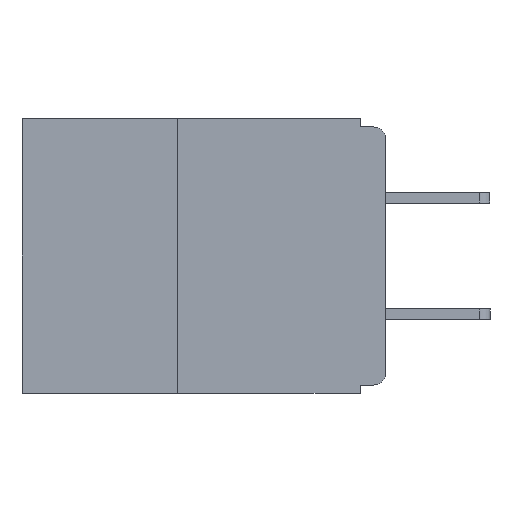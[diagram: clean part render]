
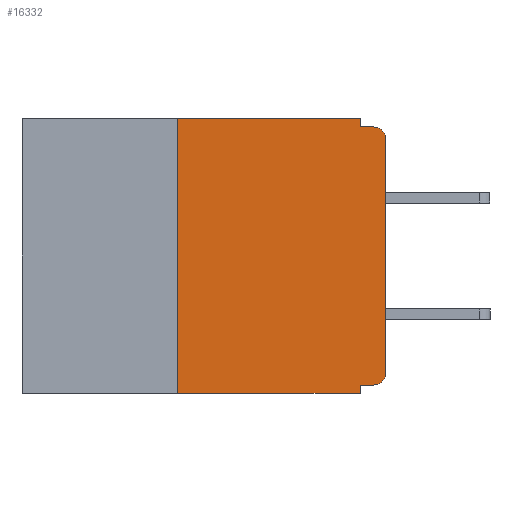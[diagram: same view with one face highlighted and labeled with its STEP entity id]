
A CAD part, left-side view. The second image highlights one B-rep face of the part: STEP entity #16332.
In plain terms, the highlighted planar face has unit normal (-1, 0, 0).
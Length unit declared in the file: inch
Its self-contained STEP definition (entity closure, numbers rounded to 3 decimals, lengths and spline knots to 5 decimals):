
#47 = VERTEX_POINT ( 'NONE', #5256 ) ;
#73 = VECTOR ( 'NONE', #1274, 39.37008 ) ;
#416 = ORIENTED_EDGE ( 'NONE', *, *, #1629, .F. ) ;
#909 = EDGE_CURVE ( 'NONE', #18240, #13265, #12853, .T. ) ;
#1192 = DIRECTION ( 'NONE',  ( 0., 0., 1. ) ) ;
#1197 = VERTEX_POINT ( 'NONE', #9864 ) ;
#1203 = LINE ( 'NONE', #15534, #5566 ) ;
#1274 = DIRECTION ( 'NONE',  ( 0., 0., -1. ) ) ;
#1463 = DIRECTION ( 'NONE',  ( 0., 0., -1. ) ) ;
#1629 = EDGE_CURVE ( 'NONE', #2551, #6083, #1203, .T. ) ;
#1816 = CARTESIAN_POINT ( 'NONE',  ( 0., 0.031, 0. ) ) ;
#2259 = CARTESIAN_POINT ( 'NONE',  ( 0., 0.437, 0. ) ) ;
#2526 = CARTESIAN_POINT ( 'NONE',  ( 0., 0.437, -0.33 ) ) ;
#2551 = VERTEX_POINT ( 'NONE', #12666 ) ;
#2767 = ORIENTED_EDGE ( 'NONE', *, *, #18670, .F. ) ;
#2886 = VECTOR ( 'NONE', #13590, 39.37008 ) ;
#2897 = CARTESIAN_POINT ( 'NONE',  ( 0., 0., 0. ) ) ;
#3027 = DIRECTION ( 'NONE',  ( -1., 0., 0. ) ) ;
#3041 = ORIENTED_EDGE ( 'NONE', *, *, #909, .F. ) ;
#3880 = EDGE_CURVE ( 'NONE', #14055, #14395, #18166, .T. ) ;
#3926 = DIRECTION ( 'NONE',  ( 0., 0., -1. ) ) ;
#4082 = CARTESIAN_POINT ( 'NONE',  ( 0., 0.437, 0. ) ) ;
#4648 = CARTESIAN_POINT ( 'NONE',  ( 0., 0.015, -0.025 ) ) ;
#4887 = AXIS2_PLACEMENT_3D ( 'NONE', #2259, #13332, #3926 ) ;
#5198 = EDGE_LOOP ( 'NONE', ( #14448, #10715, #2767, #12185, #20731, #416, #17470, #3041, #16209, #5558 ) ) ;
#5256 = CARTESIAN_POINT ( 'NONE',  ( 0., 0., -0.305 ) ) ;
#5280 = CARTESIAN_POINT ( 'NONE',  ( 0., 0., -0.01 ) ) ;
#5324 = EDGE_CURVE ( 'NONE', #2551, #13265, #7125, .T. ) ;
#5431 = LINE ( 'NONE', #2897, #16574 ) ;
#5490 = VECTOR ( 'NONE', #1463, 39.37008 ) ;
#5558 = ORIENTED_EDGE ( 'NONE', *, *, #18409, .T. ) ;
#5566 = VECTOR ( 'NONE', #15554, 39.37008 ) ;
#5738 = CARTESIAN_POINT ( 'NONE',  ( 0., 0.015, -0.32 ) ) ;
#5765 = CARTESIAN_POINT ( 'NONE',  ( 0., 0.031, -0.32 ) ) ;
#5852 = FACE_OUTER_BOUND ( 'NONE', #5198, .T. ) ;
#6083 = VERTEX_POINT ( 'NONE', #15545 ) ;
#6241 = DIRECTION ( 'NONE',  ( 0., 0., -1. ) ) ;
#6377 = VECTOR ( 'NONE', #20636, 39.37008 ) ;
#6525 = AXIS2_PLACEMENT_3D ( 'NONE', #4648, #15711, #6241 ) ;
#7125 = LINE ( 'NONE', #2526, #2886 ) ;
#8442 = DIRECTION ( 'NONE',  ( 0., -1., 0. ) ) ;
#9452 = CIRCLE ( 'NONE', #6525, 0.015 ) ;
#9468 = EDGE_CURVE ( 'NONE', #17992, #1197, #9452, .T. ) ;
#9864 = CARTESIAN_POINT ( 'NONE',  ( 0., 0.015, -0.01 ) ) ;
#10715 = ORIENTED_EDGE ( 'NONE', *, *, #9468, .T. ) ;
#10950 = CARTESIAN_POINT ( 'NONE',  ( 0., 0.031, -0.33 ) ) ;
#11063 = CARTESIAN_POINT ( 'NONE',  ( 0., 0., -0.32 ) ) ;
#12185 = ORIENTED_EDGE ( 'NONE', *, *, #3880, .F. ) ;
#12259 = CARTESIAN_POINT ( 'NONE',  ( 0., 0.031, -0.01 ) ) ;
#12495 = CARTESIAN_POINT ( 'NONE',  ( 0., 0.015, -0.305 ) ) ;
#12666 = CARTESIAN_POINT ( 'NONE',  ( 0., 0.25, -0.33 ) ) ;
#12853 = LINE ( 'NONE', #16391, #73 ) ;
#12930 = VECTOR ( 'NONE', #16735, 39.37008 ) ;
#13131 = VECTOR ( 'NONE', #8442, 39.37008 ) ;
#13265 = VERTEX_POINT ( 'NONE', #10950 ) ;
#13332 = DIRECTION ( 'NONE',  ( 1., 0., 0. ) ) ;
#13590 = DIRECTION ( 'NONE',  ( 0., -1., 0. ) ) ;
#14055 = VERTEX_POINT ( 'NONE', #19525 ) ;
#14105 = DIRECTION ( 'NONE',  ( 0., 0., -1. ) ) ;
#14310 = VERTEX_POINT ( 'NONE', #5738 ) ;
#14395 = VERTEX_POINT ( 'NONE', #12259 ) ;
#14448 = ORIENTED_EDGE ( 'NONE', *, *, #15033, .T. ) ;
#14848 = AXIS2_PLACEMENT_3D ( 'NONE', #12495, #3027, #14105 ) ;
#15033 = EDGE_CURVE ( 'NONE', #47, #17992, #5431, .T. ) ;
#15534 = CARTESIAN_POINT ( 'NONE',  ( 0., 0.25, -0.33 ) ) ;
#15545 = CARTESIAN_POINT ( 'NONE',  ( 0., 0.25, 0. ) ) ;
#15554 = DIRECTION ( 'NONE',  ( 0., 0., 1. ) ) ;
#15711 = DIRECTION ( 'NONE',  ( -1., 0., 0. ) ) ;
#15836 = EDGE_CURVE ( 'NONE', #14310, #18240, #19057, .T. ) ;
#16209 = ORIENTED_EDGE ( 'NONE', *, *, #15836, .F. ) ;
#16332 = ADVANCED_FACE ( 'NONE', ( #5852 ), #19688, .F. ) ;
#16391 = CARTESIAN_POINT ( 'NONE',  ( 0., 0.031, -0.33 ) ) ;
#16574 = VECTOR ( 'NONE', #1192, 39.37008 ) ;
#16735 = DIRECTION ( 'NONE',  ( 0., -1., 0. ) ) ;
#17217 = LINE ( 'NONE', #4082, #12930 ) ;
#17436 = LINE ( 'NONE', #5280, #13131 ) ;
#17470 = ORIENTED_EDGE ( 'NONE', *, *, #5324, .T. ) ;
#17580 = EDGE_CURVE ( 'NONE', #6083, #14055, #17217, .T. ) ;
#17992 = VERTEX_POINT ( 'NONE', #19419 ) ;
#18166 = LINE ( 'NONE', #1816, #5490 ) ;
#18208 = CIRCLE ( 'NONE', #14848, 0.015 ) ;
#18240 = VERTEX_POINT ( 'NONE', #5765 ) ;
#18409 = EDGE_CURVE ( 'NONE', #14310, #47, #18208, .T. ) ;
#18670 = EDGE_CURVE ( 'NONE', #14395, #1197, #17436, .T. ) ;
#19057 = LINE ( 'NONE', #11063, #6377 ) ;
#19419 = CARTESIAN_POINT ( 'NONE',  ( 0., 0., -0.025 ) ) ;
#19525 = CARTESIAN_POINT ( 'NONE',  ( 0., 0.031, 0. ) ) ;
#19688 = PLANE ( 'NONE',  #4887 ) ;
#20636 = DIRECTION ( 'NONE',  ( 0., 1., 0. ) ) ;
#20731 = ORIENTED_EDGE ( 'NONE', *, *, #17580, .F. ) ;
